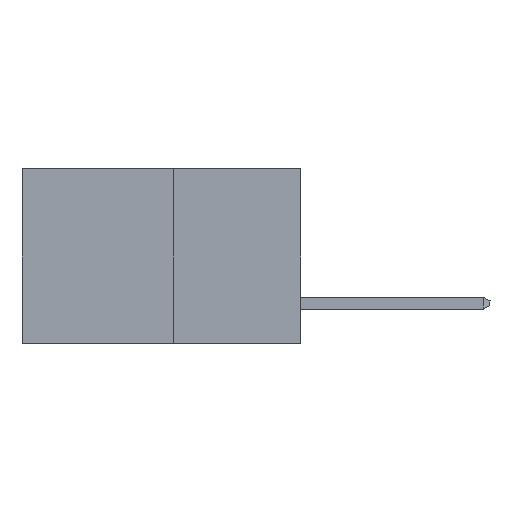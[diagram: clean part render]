
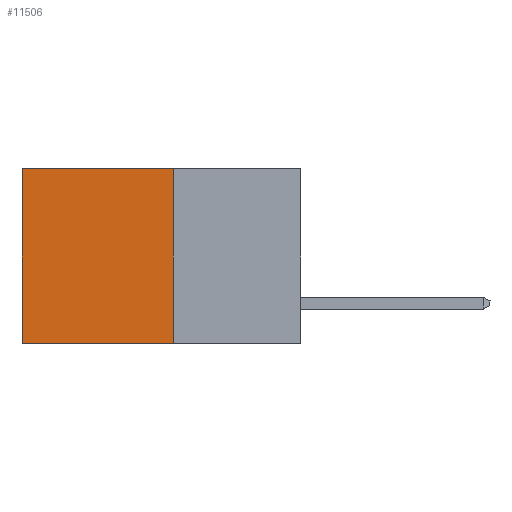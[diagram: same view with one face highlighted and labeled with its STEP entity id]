
A CAD part, left-side view. The second image highlights one B-rep face of the part: STEP entity #11506.
In plain terms, the highlighted planar face has unit normal (-1, 0, 0).
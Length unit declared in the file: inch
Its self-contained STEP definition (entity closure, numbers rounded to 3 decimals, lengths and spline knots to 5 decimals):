
#442 = LINE ( 'NONE', #6416, #5368 ) ;
#757 = DIRECTION ( 'NONE',  ( 0., 0., -1. ) ) ;
#1485 = EDGE_CURVE ( 'NONE', #6512, #6603, #11249, .T. ) ;
#1976 = VECTOR ( 'NONE', #8734, 39.37008 ) ;
#2176 = CARTESIAN_POINT ( 'NONE',  ( 0.277, 0.27, 0. ) ) ;
#2277 = VECTOR ( 'NONE', #9680, 39.37008 ) ;
#3053 = CARTESIAN_POINT ( 'NONE',  ( 0.277, 0.59, -0.37 ) ) ;
#3731 = CARTESIAN_POINT ( 'NONE',  ( 0.277, 0.27, -0.37 ) ) ;
#4053 = VERTEX_POINT ( 'NONE', #11300 ) ;
#4516 = LINE ( 'NONE', #2176, #11453 ) ;
#4823 = EDGE_LOOP ( 'NONE', ( #6190, #6199, #6235, #6269 ) ) ;
#4937 = FACE_OUTER_BOUND ( 'NONE', #4823, .T. ) ;
#5368 = VECTOR ( 'NONE', #11332, 39.37008 ) ;
#5850 = EDGE_CURVE ( 'NONE', #4053, #6603, #9445, .T. ) ;
#5888 = CARTESIAN_POINT ( 'NONE',  ( 0.277, 0.27, -0.37 ) ) ;
#6190 = ORIENTED_EDGE ( 'NONE', *, *, #5850, .T. ) ;
#6199 = ORIENTED_EDGE ( 'NONE', *, *, #1485, .F. ) ;
#6235 = ORIENTED_EDGE ( 'NONE', *, *, #10622, .F. ) ;
#6269 = ORIENTED_EDGE ( 'NONE', *, *, #10155, .T. ) ;
#6416 = CARTESIAN_POINT ( 'NONE',  ( 0.277, 0.27, -0.37 ) ) ;
#6480 = DIRECTION ( 'NONE',  ( 1., 0., 0. ) ) ;
#6512 = VERTEX_POINT ( 'NONE', #5888 ) ;
#6603 = VERTEX_POINT ( 'NONE', #3053 ) ;
#8585 = DIRECTION ( 'NONE',  ( 0., 1., 0. ) ) ;
#8734 = DIRECTION ( 'NONE',  ( 0., 1., 0. ) ) ;
#9039 = CARTESIAN_POINT ( 'NONE',  ( 0.277, 0.27, -0.37 ) ) ;
#9272 = VERTEX_POINT ( 'NONE', #9725 ) ;
#9357 = CARTESIAN_POINT ( 'NONE',  ( 0.277, 0.59, -0.37 ) ) ;
#9445 = LINE ( 'NONE', #9357, #2277 ) ;
#9680 = DIRECTION ( 'NONE',  ( 0., 0., -1. ) ) ;
#9725 = CARTESIAN_POINT ( 'NONE',  ( 0.277, 0.27, 0. ) ) ;
#10155 = EDGE_CURVE ( 'NONE', #9272, #4053, #4516, .T. ) ;
#10431 = AXIS2_PLACEMENT_3D ( 'NONE', #9039, #6480, #757 ) ;
#10622 = EDGE_CURVE ( 'NONE', #9272, #6512, #442, .T. ) ;
#11249 = LINE ( 'NONE', #3731, #1976 ) ;
#11300 = CARTESIAN_POINT ( 'NONE',  ( 0.277, 0.59, 0. ) ) ;
#11332 = DIRECTION ( 'NONE',  ( 0., 0., -1. ) ) ;
#11388 = PLANE ( 'NONE',  #10431 ) ;
#11453 = VECTOR ( 'NONE', #8585, 39.37008 ) ;
#11506 = ADVANCED_FACE ( 'NONE', ( #4937 ), #11388, .F. ) ;
